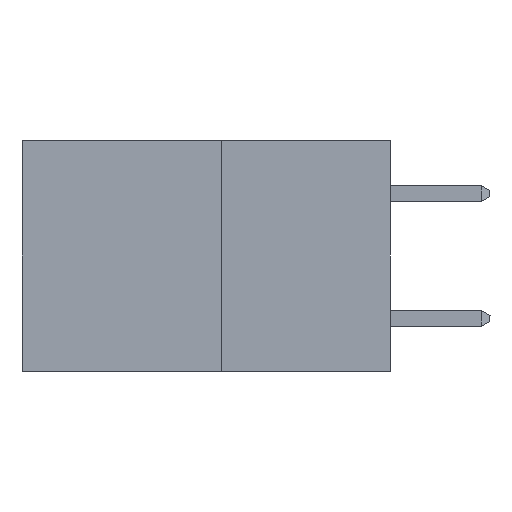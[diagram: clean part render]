
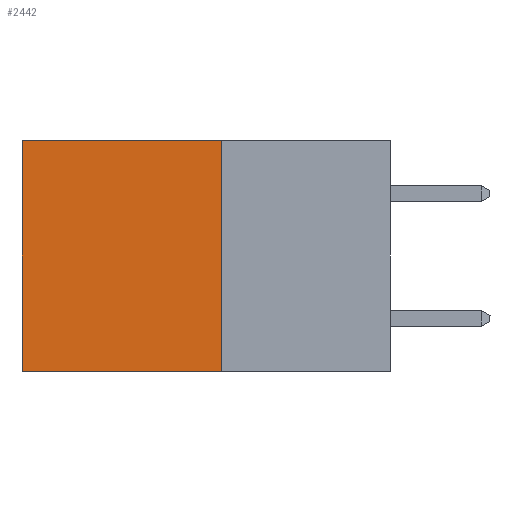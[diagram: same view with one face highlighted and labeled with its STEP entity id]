
A CAD part, left-side view. The second image highlights one B-rep face of the part: STEP entity #2442.
In plain terms, the highlighted planar face has unit normal (-1, 0, 0).
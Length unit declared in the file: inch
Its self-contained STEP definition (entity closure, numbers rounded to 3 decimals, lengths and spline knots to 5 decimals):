
#253 = DIRECTION ( 'NONE',  ( 0., 1., 0. ) ) ;
#397 = CARTESIAN_POINT ( 'NONE',  ( 0.277, 0.27, 0. ) ) ;
#583 = LINE ( 'NONE', #10257, #5195 ) ;
#1359 = AXIS2_PLACEMENT_3D ( 'NONE', #9410, #10266, #5106 ) ;
#1477 = DIRECTION ( 'NONE',  ( 0., 0., -1. ) ) ;
#1833 = VERTEX_POINT ( 'NONE', #3002 ) ;
#1974 = EDGE_CURVE ( 'NONE', #7875, #10270, #2087, .T. ) ;
#2087 = LINE ( 'NONE', #397, #11353 ) ;
#2442 = ADVANCED_FACE ( 'NONE', ( #9639 ), #3318, .F. ) ;
#2443 = EDGE_CURVE ( 'NONE', #10270, #1833, #7105, .T. ) ;
#2814 = CARTESIAN_POINT ( 'NONE',  ( 0.277, 0.59, 0. ) ) ;
#3002 = CARTESIAN_POINT ( 'NONE',  ( 0.277, 0.59, -0.37 ) ) ;
#3318 = PLANE ( 'NONE',  #1359 ) ;
#4541 = CARTESIAN_POINT ( 'NONE',  ( 0.277, 0.27, 0. ) ) ;
#5046 = VECTOR ( 'NONE', #1477, 39.37008 ) ;
#5106 = DIRECTION ( 'NONE',  ( 0., 0., -1. ) ) ;
#5195 = VECTOR ( 'NONE', #11092, 39.37008 ) ;
#5418 = CARTESIAN_POINT ( 'NONE',  ( 0.277, 0.27, -0.37 ) ) ;
#5840 = VECTOR ( 'NONE', #10229, 39.37008 ) ;
#6876 = CARTESIAN_POINT ( 'NONE',  ( 0.277, 0.59, -0.37 ) ) ;
#7105 = LINE ( 'NONE', #6876, #5046 ) ;
#7578 = EDGE_CURVE ( 'NONE', #7881, #1833, #583, .T. ) ;
#7875 = VERTEX_POINT ( 'NONE', #4541 ) ;
#7881 = VERTEX_POINT ( 'NONE', #5418 ) ;
#8186 = LINE ( 'NONE', #9376, #5840 ) ;
#9376 = CARTESIAN_POINT ( 'NONE',  ( 0.277, 0.27, -0.37 ) ) ;
#9410 = CARTESIAN_POINT ( 'NONE',  ( 0.277, 0.27, -0.37 ) ) ;
#9639 = FACE_OUTER_BOUND ( 'NONE', #11182, .T. ) ;
#9829 = EDGE_CURVE ( 'NONE', #7875, #7881, #8186, .T. ) ;
#10229 = DIRECTION ( 'NONE',  ( 0., 0., -1. ) ) ;
#10257 = CARTESIAN_POINT ( 'NONE',  ( 0.277, 0.27, -0.37 ) ) ;
#10266 = DIRECTION ( 'NONE',  ( 1., 0., 0. ) ) ;
#10270 = VERTEX_POINT ( 'NONE', #2814 ) ;
#11022 = ORIENTED_EDGE ( 'NONE', *, *, #2443, .T. ) ;
#11092 = DIRECTION ( 'NONE',  ( 0., 1., 0. ) ) ;
#11148 = ORIENTED_EDGE ( 'NONE', *, *, #7578, .F. ) ;
#11182 = EDGE_LOOP ( 'NONE', ( #11022, #11148, #11380, #11520 ) ) ;
#11353 = VECTOR ( 'NONE', #253, 39.37008 ) ;
#11380 = ORIENTED_EDGE ( 'NONE', *, *, #9829, .F. ) ;
#11520 = ORIENTED_EDGE ( 'NONE', *, *, #1974, .T. ) ;
